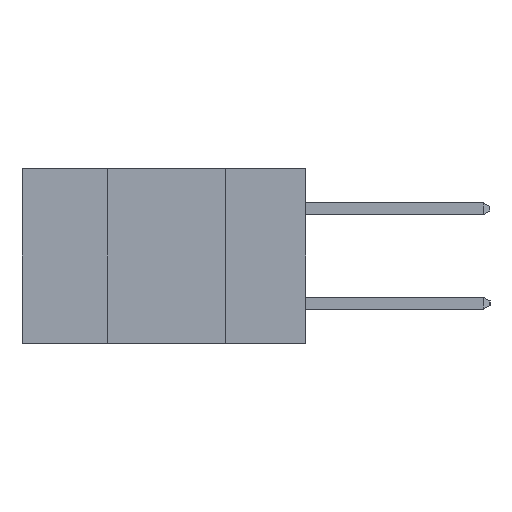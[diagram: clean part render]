
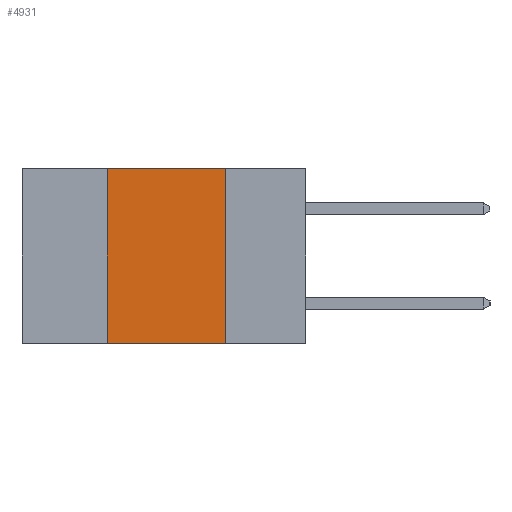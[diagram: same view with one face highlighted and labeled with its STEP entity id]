
A CAD part, left-side view. The second image highlights one B-rep face of the part: STEP entity #4931.
In plain terms, the highlighted planar face has unit normal (-1, 0, 0).
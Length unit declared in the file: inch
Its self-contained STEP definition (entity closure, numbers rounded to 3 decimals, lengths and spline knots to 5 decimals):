
#1081 = EDGE_LOOP ( 'NONE', ( #20902, #4990, #10239, #1383 ) ) ;
#1085 = CARTESIAN_POINT ( 'NONE',  ( 0., 0.42, 0. ) ) ;
#1323 = DIRECTION ( 'NONE',  ( 1., 0., 0. ) ) ;
#1383 = ORIENTED_EDGE ( 'NONE', *, *, #15583, .T. ) ;
#3804 = LINE ( 'NONE', #7728, #12629 ) ;
#4091 = VECTOR ( 'NONE', #6875, 39.37008 ) ;
#4931 = ADVANCED_FACE ( 'NONE', ( #12977 ), #11885, .F. ) ;
#4990 = ORIENTED_EDGE ( 'NONE', *, *, #16628, .F. ) ;
#5085 = CARTESIAN_POINT ( 'NONE',  ( 0., 0.17, -0.37 ) ) ;
#6038 = EDGE_CURVE ( 'NONE', #17438, #17761, #3804, .T. ) ;
#6875 = DIRECTION ( 'NONE',  ( 0., 0., -1. ) ) ;
#7081 = VECTOR ( 'NONE', #8938, 39.37008 ) ;
#7728 = CARTESIAN_POINT ( 'NONE',  ( 0., 0.42, -0.37 ) ) ;
#8938 = DIRECTION ( 'NONE',  ( 0., -1., 0. ) ) ;
#10239 = ORIENTED_EDGE ( 'NONE', *, *, #6038, .F. ) ;
#11885 = PLANE ( 'NONE',  #17905 ) ;
#12458 = VECTOR ( 'NONE', #15999, 39.37008 ) ;
#12629 = VECTOR ( 'NONE', #13014, 39.37008 ) ;
#12977 = FACE_OUTER_BOUND ( 'NONE', #1081, .T. ) ;
#13014 = DIRECTION ( 'NONE',  ( 0., 0., 1. ) ) ;
#13678 = DIRECTION ( 'NONE',  ( 0., 0., -1. ) ) ;
#13938 = CARTESIAN_POINT ( 'NONE',  ( 0., 0.17, -0.37 ) ) ;
#14255 = CARTESIAN_POINT ( 'NONE',  ( 0., 0.6, -0.37 ) ) ;
#14362 = CARTESIAN_POINT ( 'NONE',  ( 0., 0.42, -0.37 ) ) ;
#15583 = EDGE_CURVE ( 'NONE', #17438, #21303, #17137, .T. ) ;
#15920 = CARTESIAN_POINT ( 'NONE',  ( 0., 0.6, 0. ) ) ;
#15999 = DIRECTION ( 'NONE',  ( 0., -1., 0. ) ) ;
#16628 = EDGE_CURVE ( 'NONE', #17761, #17884, #17486, .T. ) ;
#17137 = LINE ( 'NONE', #14255, #12458 ) ;
#17438 = VERTEX_POINT ( 'NONE', #14362 ) ;
#17486 = LINE ( 'NONE', #15920, #7081 ) ;
#17761 = VERTEX_POINT ( 'NONE', #1085 ) ;
#17884 = VERTEX_POINT ( 'NONE', #22484 ) ;
#17905 = AXIS2_PLACEMENT_3D ( 'NONE', #22358, #1323, #13678 ) ;
#18099 = LINE ( 'NONE', #5085, #4091 ) ;
#20902 = ORIENTED_EDGE ( 'NONE', *, *, #21271, .F. ) ;
#21271 = EDGE_CURVE ( 'NONE', #17884, #21303, #18099, .T. ) ;
#21303 = VERTEX_POINT ( 'NONE', #13938 ) ;
#22358 = CARTESIAN_POINT ( 'NONE',  ( 0., 0.6, 0. ) ) ;
#22484 = CARTESIAN_POINT ( 'NONE',  ( 0., 0.17, 0. ) ) ;
